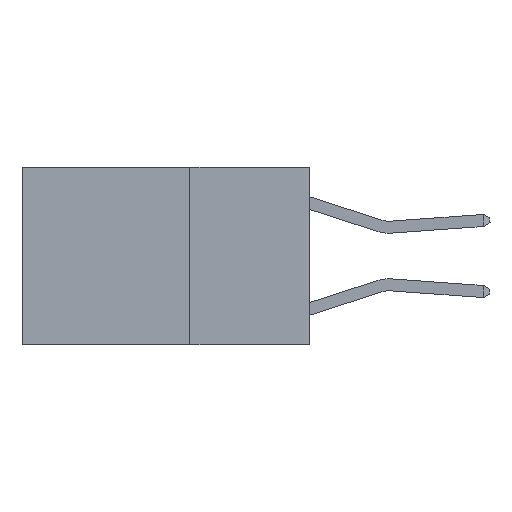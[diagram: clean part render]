
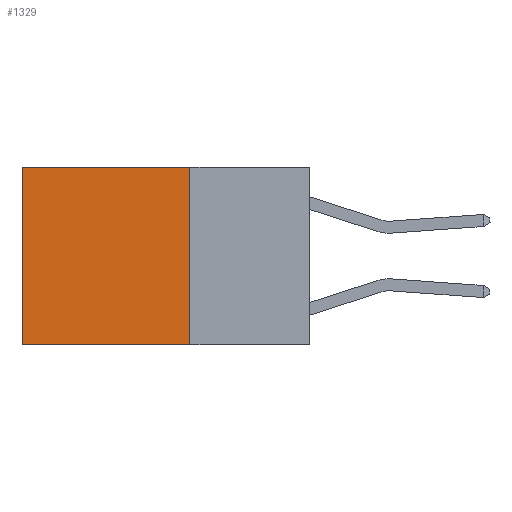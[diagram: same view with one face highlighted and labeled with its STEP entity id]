
A CAD part, left-side view. The second image highlights one B-rep face of the part: STEP entity #1329.
In plain terms, the highlighted planar face has unit normal (-1, 0, 0).
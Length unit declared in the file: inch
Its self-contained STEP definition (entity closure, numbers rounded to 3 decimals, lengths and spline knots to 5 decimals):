
#289 = CARTESIAN_POINT ( 'NONE',  ( 0.2625, 0.25, 0. ) ) ;
#539 = EDGE_LOOP ( 'NONE', ( #9749, #15978, #22182, #6831 ) ) ;
#758 = VERTEX_POINT ( 'NONE', #7244 ) ;
#1329 = ADVANCED_FACE ( 'NONE', ( #12519 ), #20186, .F. ) ;
#1389 = LINE ( 'NONE', #5149, #18942 ) ;
#1675 = DIRECTION ( 'NONE',  ( 0., 0., -1. ) ) ;
#2966 = VECTOR ( 'NONE', #16493, 39.37008 ) ;
#3666 = DIRECTION ( 'NONE',  ( 1., 0., 0. ) ) ;
#4886 = CARTESIAN_POINT ( 'NONE',  ( 0.2625, 0.6, -0.37 ) ) ;
#5003 = CARTESIAN_POINT ( 'NONE',  ( 0.2625, 0.25, 0. ) ) ;
#5149 = CARTESIAN_POINT ( 'NONE',  ( 0.2625, 0.6, 0. ) ) ;
#6216 = VECTOR ( 'NONE', #7023, 39.37008 ) ;
#6831 = ORIENTED_EDGE ( 'NONE', *, *, #21852, .T. ) ;
#7023 = DIRECTION ( 'NONE',  ( 0., 1., 0. ) ) ;
#7048 = CARTESIAN_POINT ( 'NONE',  ( 0.2625, 0.25, -0.37 ) ) ;
#7244 = CARTESIAN_POINT ( 'NONE',  ( 0.2625, 0.25, -0.37 ) ) ;
#9704 = LINE ( 'NONE', #19510, #13542 ) ;
#9749 = ORIENTED_EDGE ( 'NONE', *, *, #18840, .T. ) ;
#9786 = CARTESIAN_POINT ( 'NONE',  ( 0.2625, 0.6, 0. ) ) ;
#12519 = FACE_OUTER_BOUND ( 'NONE', #539, .T. ) ;
#13542 = VECTOR ( 'NONE', #19259, 39.37008 ) ;
#14421 = EDGE_CURVE ( 'NONE', #758, #23496, #20754, .T. ) ;
#15013 = CARTESIAN_POINT ( 'NONE',  ( 0.2625, 0.25, 0. ) ) ;
#15070 = LINE ( 'NONE', #5003, #6216 ) ;
#15169 = AXIS2_PLACEMENT_3D ( 'NONE', #15013, #3666, #1675 ) ;
#15978 = ORIENTED_EDGE ( 'NONE', *, *, #14421, .F. ) ;
#16493 = DIRECTION ( 'NONE',  ( 0., 1., 0. ) ) ;
#17403 = EDGE_CURVE ( 'NONE', #22420, #758, #9704, .T. ) ;
#18840 = EDGE_CURVE ( 'NONE', #21954, #23496, #1389, .T. ) ;
#18942 = VECTOR ( 'NONE', #20880, 39.37008 ) ;
#19259 = DIRECTION ( 'NONE',  ( 0., 0., -1. ) ) ;
#19510 = CARTESIAN_POINT ( 'NONE',  ( 0.2625, 0.25, 0. ) ) ;
#20186 = PLANE ( 'NONE',  #15169 ) ;
#20754 = LINE ( 'NONE', #7048, #2966 ) ;
#20880 = DIRECTION ( 'NONE',  ( 0., 0., -1. ) ) ;
#21852 = EDGE_CURVE ( 'NONE', #22420, #21954, #15070, .T. ) ;
#21954 = VERTEX_POINT ( 'NONE', #9786 ) ;
#22182 = ORIENTED_EDGE ( 'NONE', *, *, #17403, .F. ) ;
#22420 = VERTEX_POINT ( 'NONE', #289 ) ;
#23496 = VERTEX_POINT ( 'NONE', #4886 ) ;
